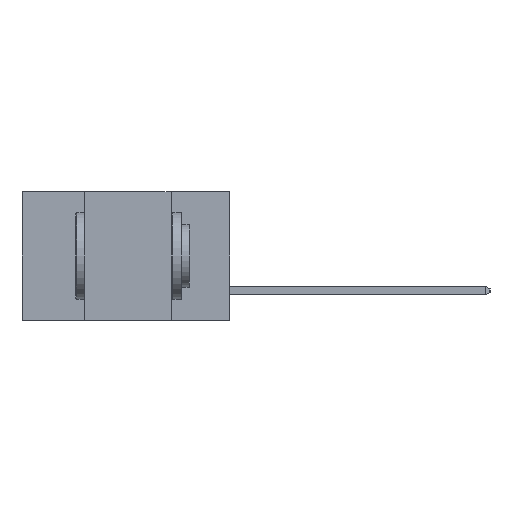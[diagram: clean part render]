
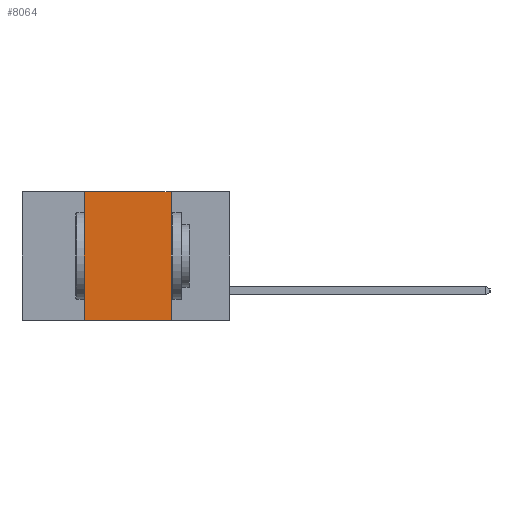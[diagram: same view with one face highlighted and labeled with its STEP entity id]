
A CAD part, left-side view. The second image highlights one B-rep face of the part: STEP entity #8064.
In plain terms, the highlighted planar face has unit normal (-1, 0, 0).
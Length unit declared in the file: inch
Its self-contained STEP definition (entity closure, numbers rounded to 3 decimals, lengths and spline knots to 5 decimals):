
#238 = CARTESIAN_POINT ( 'NONE',  ( 0., 0.6, 0. ) ) ;
#349 = VERTEX_POINT ( 'NONE', #11154 ) ;
#1044 = CARTESIAN_POINT ( 'NONE',  ( 0., 0.17, -0.37 ) ) ;
#1252 = VERTEX_POINT ( 'NONE', #9565 ) ;
#1275 = VECTOR ( 'NONE', #2299, 39.37008 ) ;
#1426 = DIRECTION ( 'NONE',  ( 0., 0., -1. ) ) ;
#1901 = VECTOR ( 'NONE', #6406, 39.37008 ) ;
#2084 = DIRECTION ( 'NONE',  ( 0., -1., 0. ) ) ;
#2299 = DIRECTION ( 'NONE',  ( 0., 0., 1. ) ) ;
#2684 = LINE ( 'NONE', #10607, #4797 ) ;
#2982 = CARTESIAN_POINT ( 'NONE',  ( 0., 0.17, 0. ) ) ;
#3222 = VERTEX_POINT ( 'NONE', #1044 ) ;
#4797 = VECTOR ( 'NONE', #2084, 39.37008 ) ;
#5520 = FACE_OUTER_BOUND ( 'NONE', #6500, .T. ) ;
#6155 = VERTEX_POINT ( 'NONE', #11582 ) ;
#6406 = DIRECTION ( 'NONE',  ( 0., -1., 0. ) ) ;
#6500 = EDGE_LOOP ( 'NONE', ( #7789, #10938, #7943, #8317 ) ) ;
#6708 = EDGE_CURVE ( 'NONE', #6155, #3222, #2684, .T. ) ;
#7148 = EDGE_CURVE ( 'NONE', #349, #1252, #14671, .T. ) ;
#7212 = CARTESIAN_POINT ( 'NONE',  ( 0., 0.42, 0. ) ) ;
#7789 = ORIENTED_EDGE ( 'NONE', *, *, #11537, .F. ) ;
#7943 = ORIENTED_EDGE ( 'NONE', *, *, #9175, .F. ) ;
#7952 = DIRECTION ( 'NONE',  ( 0., 0., -1. ) ) ;
#8064 = ADVANCED_FACE ( 'NONE', ( #5520 ), #8737, .F. ) ;
#8317 = ORIENTED_EDGE ( 'NONE', *, *, #6708, .T. ) ;
#8737 = PLANE ( 'NONE',  #8892 ) ;
#8776 = VECTOR ( 'NONE', #7952, 39.37008 ) ;
#8783 = DIRECTION ( 'NONE',  ( 1., 0., 0. ) ) ;
#8892 = AXIS2_PLACEMENT_3D ( 'NONE', #238, #8783, #1426 ) ;
#9175 = EDGE_CURVE ( 'NONE', #6155, #349, #10983, .T. ) ;
#9565 = CARTESIAN_POINT ( 'NONE',  ( 0., 0.17, 0. ) ) ;
#10607 = CARTESIAN_POINT ( 'NONE',  ( 0., 0.6, -0.37 ) ) ;
#10938 = ORIENTED_EDGE ( 'NONE', *, *, #7148, .F. ) ;
#10983 = LINE ( 'NONE', #7212, #1275 ) ;
#11154 = CARTESIAN_POINT ( 'NONE',  ( 0., 0.42, 0. ) ) ;
#11537 = EDGE_CURVE ( 'NONE', #1252, #3222, #11908, .T. ) ;
#11582 = CARTESIAN_POINT ( 'NONE',  ( 0., 0.42, -0.37 ) ) ;
#11908 = LINE ( 'NONE', #2982, #8776 ) ;
#13689 = CARTESIAN_POINT ( 'NONE',  ( 0., 0.6, 0. ) ) ;
#14671 = LINE ( 'NONE', #13689, #1901 ) ;
